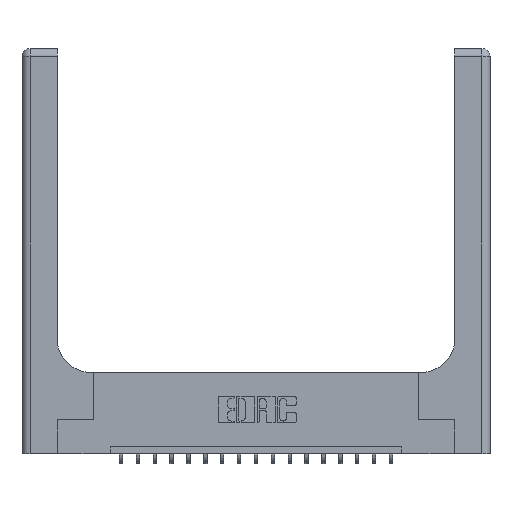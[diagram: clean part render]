
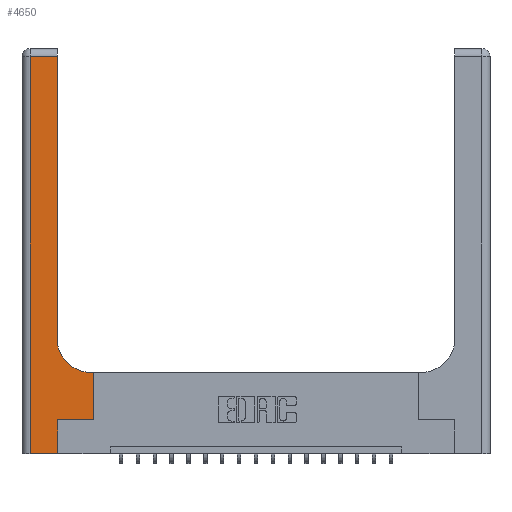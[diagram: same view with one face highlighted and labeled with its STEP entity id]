
A CAD part, top view. The second image highlights one B-rep face of the part: STEP entity #4650.
In plain terms, the highlighted planar face has unit normal (0, 0, 1).
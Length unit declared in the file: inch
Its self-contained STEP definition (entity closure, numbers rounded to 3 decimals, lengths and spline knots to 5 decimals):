
#68 = VERTEX_POINT ( 'NONE', #17974 ) ;
#384 = CARTESIAN_POINT ( 'NONE',  ( 0.06, 2.94, 0.37 ) ) ;
#534 = DIRECTION ( 'NONE',  ( -1., 0., 0. ) ) ;
#1178 = EDGE_CURVE ( 'NONE', #4603, #5606, #4020, .T. ) ;
#1181 = CARTESIAN_POINT ( 'NONE',  ( 0., 2.94, 0.37 ) ) ;
#1455 = EDGE_CURVE ( 'NONE', #68, #10584, #15060, .T. ) ;
#1626 = EDGE_LOOP ( 'NONE', ( #3461, #12205, #17565, #16421, #7933, #11771, #1844, #9737, #18967 ) ) ;
#1674 = CARTESIAN_POINT ( 'NONE',  ( 0.265, 0.25, 0.37 ) ) ;
#1844 = ORIENTED_EDGE ( 'NONE', *, *, #1178, .T. ) ;
#2260 = CARTESIAN_POINT ( 'NONE',  ( 0., 3., 0.37 ) ) ;
#2565 = EDGE_CURVE ( 'NONE', #10584, #14796, #9962, .T. ) ;
#2574 = LINE ( 'NONE', #11842, #13881 ) ;
#2600 = LINE ( 'NONE', #5847, #6603 ) ;
#2798 = DIRECTION ( 'NONE',  ( 0., 1., 0. ) ) ;
#2984 = AXIS2_PLACEMENT_3D ( 'NONE', #15234, #6467, #16750 ) ;
#3143 = AXIS2_PLACEMENT_3D ( 'NONE', #2260, #18618, #9784 ) ;
#3461 = ORIENTED_EDGE ( 'NONE', *, *, #2565, .T. ) ;
#3743 = CARTESIAN_POINT ( 'NONE',  ( 0.265, 0., 0.37 ) ) ;
#4020 = LINE ( 'NONE', #10245, #18788 ) ;
#4603 = VERTEX_POINT ( 'NONE', #6722 ) ;
#4650 = ADVANCED_FACE ( 'NONE', ( #15183 ), #8333, .F. ) ;
#4793 = LINE ( 'NONE', #10944, #8737 ) ;
#5317 = LINE ( 'NONE', #16456, #12644 ) ;
#5606 = VERTEX_POINT ( 'NONE', #10594 ) ;
#5847 = CARTESIAN_POINT ( 'NONE',  ( 0.06, 3., 0.37 ) ) ;
#6467 = DIRECTION ( 'NONE',  ( 0., 0., -1. ) ) ;
#6523 = CARTESIAN_POINT ( 'NONE',  ( 0.26, 0.85, 0.37 ) ) ;
#6603 = VECTOR ( 'NONE', #7363, 39.37008 ) ;
#6722 = CARTESIAN_POINT ( 'NONE',  ( 0.528, 0.25, 0.37 ) ) ;
#7363 = DIRECTION ( 'NONE',  ( 0., -1., 0. ) ) ;
#7484 = LINE ( 'NONE', #7511, #18736 ) ;
#7511 = CARTESIAN_POINT ( 'NONE',  ( 0., 0., 0.37 ) ) ;
#7857 = DIRECTION ( 'NONE',  ( 0., 1., 0. ) ) ;
#7933 = ORIENTED_EDGE ( 'NONE', *, *, #13704, .T. ) ;
#8333 = PLANE ( 'NONE',  #3143 ) ;
#8737 = VECTOR ( 'NONE', #534, 39.37008 ) ;
#9737 = ORIENTED_EDGE ( 'NONE', *, *, #16866, .T. ) ;
#9784 = DIRECTION ( 'NONE',  ( -1., 0., 0. ) ) ;
#9962 = LINE ( 'NONE', #10719, #17812 ) ;
#10245 = CARTESIAN_POINT ( 'NONE',  ( 0.528, 0.25, 0.37 ) ) ;
#10405 = EDGE_CURVE ( 'NONE', #16767, #19082, #7484, .T. ) ;
#10584 = VERTEX_POINT ( 'NONE', #6523 ) ;
#10594 = CARTESIAN_POINT ( 'NONE',  ( 0.528, 0.6, 0.37 ) ) ;
#10719 = CARTESIAN_POINT ( 'NONE',  ( 0.26, 3., 0.37 ) ) ;
#10944 = CARTESIAN_POINT ( 'NONE',  ( 0.26, 0.6, 0.37 ) ) ;
#10974 = VECTOR ( 'NONE', #18978, 39.37008 ) ;
#11418 = LINE ( 'NONE', #1181, #10974 ) ;
#11771 = ORIENTED_EDGE ( 'NONE', *, *, #15441, .T. ) ;
#11842 = CARTESIAN_POINT ( 'NONE',  ( 0.265, 0., 0.37 ) ) ;
#12136 = CARTESIAN_POINT ( 'NONE',  ( 0.06, 0., 0.37 ) ) ;
#12205 = ORIENTED_EDGE ( 'NONE', *, *, #17689, .T. ) ;
#12363 = VERTEX_POINT ( 'NONE', #1674 ) ;
#12644 = VECTOR ( 'NONE', #17937, 39.37008 ) ;
#13310 = DIRECTION ( 'NONE',  ( 0., 1., 0. ) ) ;
#13340 = CARTESIAN_POINT ( 'NONE',  ( 0.26, 2.94, 0.37 ) ) ;
#13348 = DIRECTION ( 'NONE',  ( 1., 0., 0. ) ) ;
#13704 = EDGE_CURVE ( 'NONE', #19082, #12363, #2574, .T. ) ;
#13881 = VECTOR ( 'NONE', #13310, 39.37008 ) ;
#14796 = VERTEX_POINT ( 'NONE', #13340 ) ;
#15060 = CIRCLE ( 'NONE', #2984, 0.25 ) ;
#15183 = FACE_OUTER_BOUND ( 'NONE', #1626, .T. ) ;
#15234 = CARTESIAN_POINT ( 'NONE',  ( 0.51, 0.85, 0.37 ) ) ;
#15441 = EDGE_CURVE ( 'NONE', #12363, #4603, #5317, .T. ) ;
#15568 = VERTEX_POINT ( 'NONE', #384 ) ;
#16421 = ORIENTED_EDGE ( 'NONE', *, *, #10405, .T. ) ;
#16456 = CARTESIAN_POINT ( 'NONE',  ( 0.265, 0.25, 0.37 ) ) ;
#16750 = DIRECTION ( 'NONE',  ( 1., 0., 0. ) ) ;
#16767 = VERTEX_POINT ( 'NONE', #12136 ) ;
#16866 = EDGE_CURVE ( 'NONE', #5606, #68, #4793, .T. ) ;
#17565 = ORIENTED_EDGE ( 'NONE', *, *, #18675, .T. ) ;
#17689 = EDGE_CURVE ( 'NONE', #14796, #15568, #11418, .T. ) ;
#17812 = VECTOR ( 'NONE', #7857, 39.37008 ) ;
#17937 = DIRECTION ( 'NONE',  ( 1., 0., 0. ) ) ;
#17974 = CARTESIAN_POINT ( 'NONE',  ( 0.51, 0.6, 0.37 ) ) ;
#18618 = DIRECTION ( 'NONE',  ( 0., 0., -1. ) ) ;
#18675 = EDGE_CURVE ( 'NONE', #15568, #16767, #2600, .T. ) ;
#18736 = VECTOR ( 'NONE', #13348, 39.37008 ) ;
#18788 = VECTOR ( 'NONE', #2798, 39.37008 ) ;
#18967 = ORIENTED_EDGE ( 'NONE', *, *, #1455, .T. ) ;
#18978 = DIRECTION ( 'NONE',  ( -1., 0., 0. ) ) ;
#19082 = VERTEX_POINT ( 'NONE', #3743 ) ;
